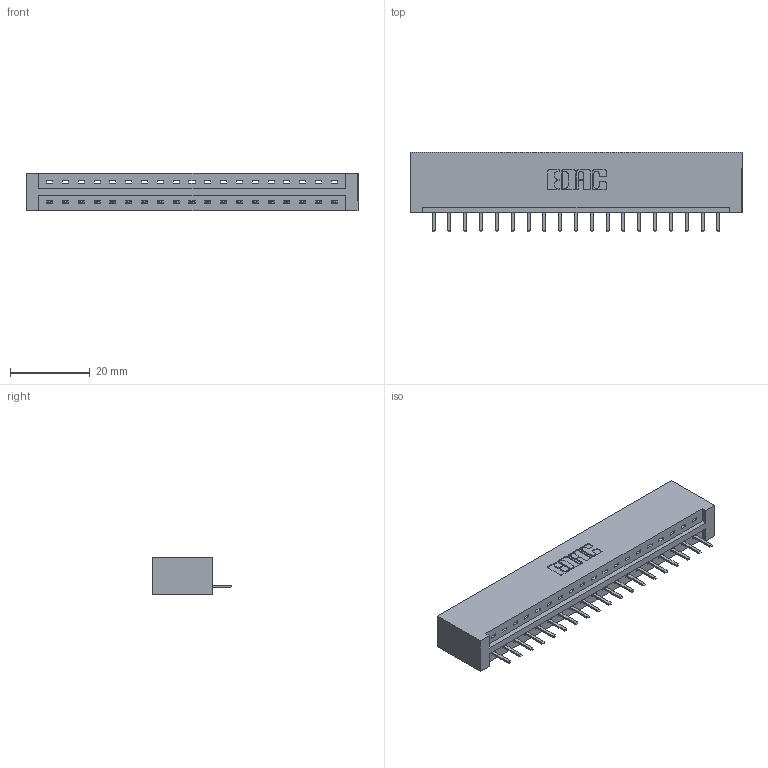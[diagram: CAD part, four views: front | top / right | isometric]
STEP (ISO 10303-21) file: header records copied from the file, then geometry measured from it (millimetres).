
FILE_DESCRIPTION (( 'STEP AP203' ), '1' );
FILE_NAME ('337-019-520-101.STEP', '2018-08-05T06:47:16', ( '' ), ( '' ), 'SwSTEP 2.0', 'SolidWorks 2016', '' );
FILE_SCHEMA (( 'CONFIG_CONTROL_DESIGN' ));
Length unit declared in the file: inch
Products named in the file (3): 337 Part_No Mounting Lugs; 345-292-001_345-293-120; 337-019-520-101
Assembly tree (20 placements, depth 2):
  337-019-520-101
    337 Part_No Mounting Lugs
    345-292-001_345-293-120  x19
Bounding box: 83.16 x 20.02 x 9.4 mm (x, y, z)
Volume: 9039.3 mm3; surface area: 8997.8 mm2
Topology: 20 solids, 20 shells, 1360 faces, 4011 edges, 2622 vertices
Faces by surface type: plane 978, cylinder 382
Entity records: 16935 total; most frequent: CARTESIAN_POINT 2967, ORIENTED_EDGE 2910, DIRECTION 2525, EDGE_CURVE 1455, VECTOR 1331, LINE 1331, VERTEX_POINT 966, AXIS2_PLACEMENT_3D 597
